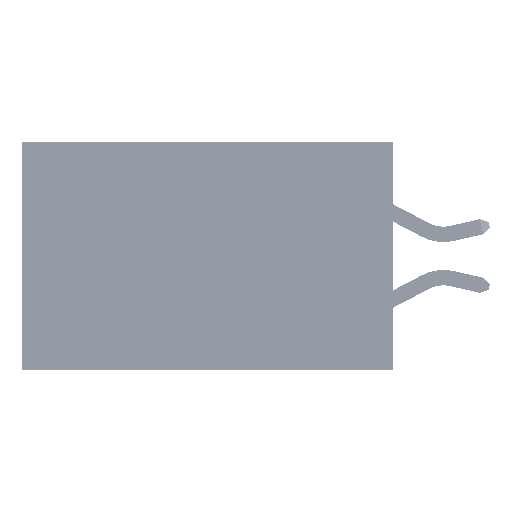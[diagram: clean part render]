
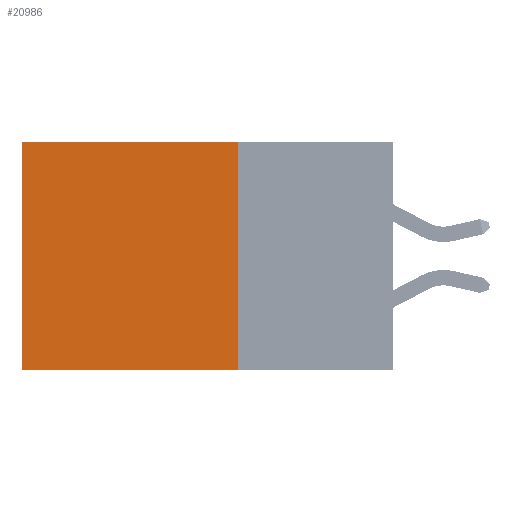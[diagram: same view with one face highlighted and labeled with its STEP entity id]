
A CAD part, left-side view. The second image highlights one B-rep face of the part: STEP entity #20986.
In plain terms, the highlighted planar face has unit normal (-1, 0, 0).
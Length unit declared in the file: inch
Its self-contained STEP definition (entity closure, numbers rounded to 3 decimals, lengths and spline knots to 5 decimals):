
#818 = DIRECTION ( 'NONE',  ( 0., 1., 0. ) ) ;
#931 = CARTESIAN_POINT ( 'NONE',  ( 0.2875, 0.6, 0. ) ) ;
#4575 = DIRECTION ( 'NONE',  ( 1., 0., 0. ) ) ;
#5094 = AXIS2_PLACEMENT_3D ( 'NONE', #29403, #4575, #32958 ) ;
#5600 = ORIENTED_EDGE ( 'NONE', *, *, #21001, .F. ) ;
#10902 = DIRECTION ( 'NONE',  ( 0., 0., -1. ) ) ;
#11221 = EDGE_LOOP ( 'NONE', ( #34358, #32199, #5600, #16895 ) ) ;
#15310 = CARTESIAN_POINT ( 'NONE',  ( 0.2875, 0.25, 0. ) ) ;
#16895 = ORIENTED_EDGE ( 'NONE', *, *, #42185, .T. ) ;
#18350 = EDGE_CURVE ( 'NONE', #19106, #19299, #24862, .T. ) ;
#18904 = CARTESIAN_POINT ( 'NONE',  ( 0.2875, 0.25, 0. ) ) ;
#19106 = VERTEX_POINT ( 'NONE', #931 ) ;
#19299 = VERTEX_POINT ( 'NONE', #23466 ) ;
#20495 = LINE ( 'NONE', #27866, #42459 ) ;
#20986 = ADVANCED_FACE ( 'NONE', ( #23200 ), #32368, .F. ) ;
#21001 = EDGE_CURVE ( 'NONE', #31215, #31568, #21556, .T. ) ;
#21393 = VECTOR ( 'NONE', #818, 39.37008 ) ;
#21556 = LINE ( 'NONE', #15310, #32524 ) ;
#23200 = FACE_OUTER_BOUND ( 'NONE', #11221, .T. ) ;
#23466 = CARTESIAN_POINT ( 'NONE',  ( 0.2875, 0.6, -0.37 ) ) ;
#24862 = LINE ( 'NONE', #28540, #38622 ) ;
#25208 = CARTESIAN_POINT ( 'NONE',  ( 0.2875, 0.25, -0.37 ) ) ;
#27866 = CARTESIAN_POINT ( 'NONE',  ( 0.2875, 0.25, 0. ) ) ;
#28540 = CARTESIAN_POINT ( 'NONE',  ( 0.2875, 0.6, 0. ) ) ;
#28948 = DIRECTION ( 'NONE',  ( 0., 0., -1. ) ) ;
#29403 = CARTESIAN_POINT ( 'NONE',  ( 0.2875, 0.25, 0. ) ) ;
#31215 = VERTEX_POINT ( 'NONE', #18904 ) ;
#31568 = VERTEX_POINT ( 'NONE', #42049 ) ;
#32199 = ORIENTED_EDGE ( 'NONE', *, *, #37429, .F. ) ;
#32368 = PLANE ( 'NONE',  #5094 ) ;
#32524 = VECTOR ( 'NONE', #28948, 39.37008 ) ;
#32923 = LINE ( 'NONE', #25208, #21393 ) ;
#32958 = DIRECTION ( 'NONE',  ( 0., 0., -1. ) ) ;
#34358 = ORIENTED_EDGE ( 'NONE', *, *, #18350, .T. ) ;
#37429 = EDGE_CURVE ( 'NONE', #31568, #19299, #32923, .T. ) ;
#38094 = DIRECTION ( 'NONE',  ( 0., 1., 0. ) ) ;
#38622 = VECTOR ( 'NONE', #10902, 39.37008 ) ;
#42049 = CARTESIAN_POINT ( 'NONE',  ( 0.2875, 0.25, -0.37 ) ) ;
#42185 = EDGE_CURVE ( 'NONE', #31215, #19106, #20495, .T. ) ;
#42459 = VECTOR ( 'NONE', #38094, 39.37008 ) ;
